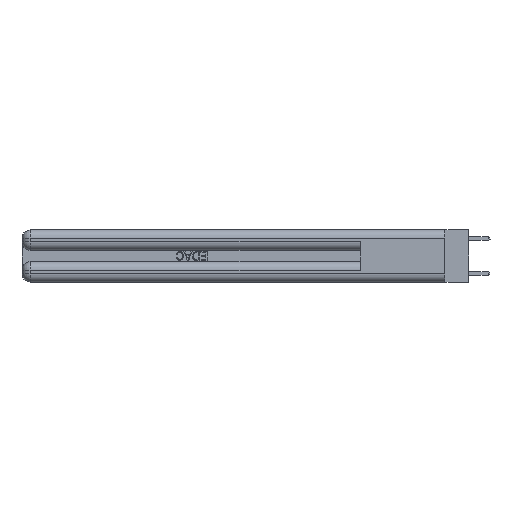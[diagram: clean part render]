
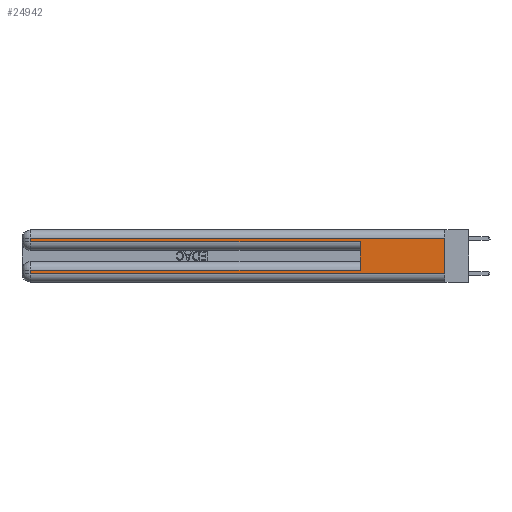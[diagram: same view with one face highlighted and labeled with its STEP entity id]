
A CAD part, left-side view. The second image highlights one B-rep face of the part: STEP entity #24942.
In plain terms, the highlighted planar face has unit normal (-1, 0, 0).
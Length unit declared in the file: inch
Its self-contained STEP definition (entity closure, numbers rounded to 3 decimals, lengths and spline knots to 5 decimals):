
#343 = CARTESIAN_POINT ( 'NONE',  ( 0., 2.94, 0.285 ) ) ;
#2008 = CARTESIAN_POINT ( 'NONE',  ( 0., 2.94, 0.06 ) ) ;
#2359 = EDGE_CURVE ( 'NONE', #29691, #16403, #27238, .T. ) ;
#2627 = FACE_OUTER_BOUND ( 'NONE', #28935, .T. ) ;
#3300 = CARTESIAN_POINT ( 'NONE',  ( 0., 0., 0.06 ) ) ;
#3423 = CARTESIAN_POINT ( 'NONE',  ( 0., 0., 0.37 ) ) ;
#3973 = CARTESIAN_POINT ( 'NONE',  ( 0., 0., 0.285 ) ) ;
#4083 = ORIENTED_EDGE ( 'NONE', *, *, #9141, .F. ) ;
#4113 = EDGE_CURVE ( 'NONE', #17205, #34553, #5240, .T. ) ;
#4207 = EDGE_CURVE ( 'NONE', #23861, #13758, #32838, .T. ) ;
#5240 = LINE ( 'NONE', #28368, #19640 ) ;
#5507 = ORIENTED_EDGE ( 'NONE', *, *, #21826, .T. ) ;
#5696 = CARTESIAN_POINT ( 'NONE',  ( 0., 2.94, 0.31 ) ) ;
#5783 = CARTESIAN_POINT ( 'NONE',  ( 0., 2.94, 0.37 ) ) ;
#6087 = ORIENTED_EDGE ( 'NONE', *, *, #4207, .T. ) ;
#6289 = DIRECTION ( 'NONE',  ( 0., -1., 0. ) ) ;
#7030 = VECTOR ( 'NONE', #23836, 39.37008 ) ;
#7808 = ORIENTED_EDGE ( 'NONE', *, *, #24113, .T. ) ;
#7898 = LINE ( 'NONE', #26539, #7030 ) ;
#9141 = EDGE_CURVE ( 'NONE', #13674, #19069, #11163, .T. ) ;
#10125 = ORIENTED_EDGE ( 'NONE', *, *, #2359, .F. ) ;
#10170 = ORIENTED_EDGE ( 'NONE', *, *, #24531, .T. ) ;
#10204 = VECTOR ( 'NONE', #25935, 39.37008 ) ;
#11163 = LINE ( 'NONE', #3423, #18797 ) ;
#11595 = ORIENTED_EDGE ( 'NONE', *, *, #4113, .T. ) ;
#12117 = VECTOR ( 'NONE', #23699, 39.37008 ) ;
#12454 = ORIENTED_EDGE ( 'NONE', *, *, #27266, .T. ) ;
#13577 = DIRECTION ( 'NONE',  ( 1., 0., 0. ) ) ;
#13674 = VERTEX_POINT ( 'NONE', #14514 ) ;
#13758 = VERTEX_POINT ( 'NONE', #343 ) ;
#14023 = VECTOR ( 'NONE', #24106, 39.37008 ) ;
#14514 = CARTESIAN_POINT ( 'NONE',  ( 0., 0., 0.31 ) ) ;
#15111 = CARTESIAN_POINT ( 'NONE',  ( 0., 0.6, 0.145 ) ) ;
#16403 = VERTEX_POINT ( 'NONE', #25468 ) ;
#17205 = VERTEX_POINT ( 'NONE', #26045 ) ;
#17567 = LINE ( 'NONE', #31663, #22449 ) ;
#17595 = DIRECTION ( 'NONE',  ( 0., 1., 0. ) ) ;
#17609 = CARTESIAN_POINT ( 'NONE',  ( 0., 0., 0.06 ) ) ;
#18797 = VECTOR ( 'NONE', #20696, 39.37008 ) ;
#19069 = VERTEX_POINT ( 'NONE', #17609 ) ;
#19073 = AXIS2_PLACEMENT_3D ( 'NONE', #30541, #13577, #33318 ) ;
#19640 = VECTOR ( 'NONE', #22836, 39.37008 ) ;
#20696 = DIRECTION ( 'NONE',  ( 0., 0., -1. ) ) ;
#21826 = EDGE_CURVE ( 'NONE', #13674, #23861, #7898, .T. ) ;
#22449 = VECTOR ( 'NONE', #17595, 39.37008 ) ;
#22539 = LINE ( 'NONE', #3300, #36505 ) ;
#22836 = DIRECTION ( 'NONE',  ( 0., 0., -1. ) ) ;
#23699 = DIRECTION ( 'NONE',  ( 0., 0., 1. ) ) ;
#23836 = DIRECTION ( 'NONE',  ( 0., 1., 0. ) ) ;
#23861 = VERTEX_POINT ( 'NONE', #5696 ) ;
#24106 = DIRECTION ( 'NONE',  ( 0., -1., 0. ) ) ;
#24113 = EDGE_CURVE ( 'NONE', #13758, #16403, #28200, .T. ) ;
#24531 = EDGE_CURVE ( 'NONE', #29691, #17205, #17567, .T. ) ;
#24942 = ADVANCED_FACE ( 'NONE', ( #2627 ), #35870, .F. ) ;
#25468 = CARTESIAN_POINT ( 'NONE',  ( 0., 0.6, 0.285 ) ) ;
#25935 = DIRECTION ( 'NONE',  ( 0., 0., -1. ) ) ;
#26045 = CARTESIAN_POINT ( 'NONE',  ( 0., 2.94, 0.085 ) ) ;
#26539 = CARTESIAN_POINT ( 'NONE',  ( 0., 0., 0.31 ) ) ;
#27238 = LINE ( 'NONE', #15111, #12117 ) ;
#27266 = EDGE_CURVE ( 'NONE', #34553, #19069, #22539, .T. ) ;
#28200 = LINE ( 'NONE', #3973, #14023 ) ;
#28368 = CARTESIAN_POINT ( 'NONE',  ( 0., 2.94, 0.37 ) ) ;
#28935 = EDGE_LOOP ( 'NONE', ( #4083, #5507, #6087, #7808, #10125, #10170, #11595, #12454 ) ) ;
#29691 = VERTEX_POINT ( 'NONE', #35161 ) ;
#30541 = CARTESIAN_POINT ( 'NONE',  ( 0., 0., 0.37 ) ) ;
#31663 = CARTESIAN_POINT ( 'NONE',  ( 0., 0., 0.085 ) ) ;
#32838 = LINE ( 'NONE', #5783, #10204 ) ;
#33318 = DIRECTION ( 'NONE',  ( 0., 0., -1. ) ) ;
#34553 = VERTEX_POINT ( 'NONE', #2008 ) ;
#35161 = CARTESIAN_POINT ( 'NONE',  ( 0., 0.6, 0.085 ) ) ;
#35870 = PLANE ( 'NONE',  #19073 ) ;
#36505 = VECTOR ( 'NONE', #6289, 39.37008 ) ;
